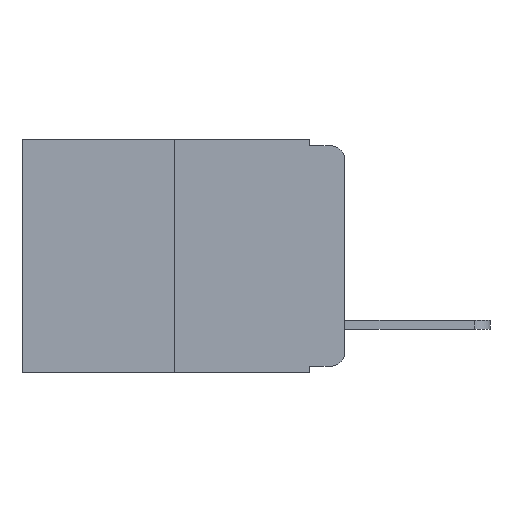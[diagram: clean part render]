
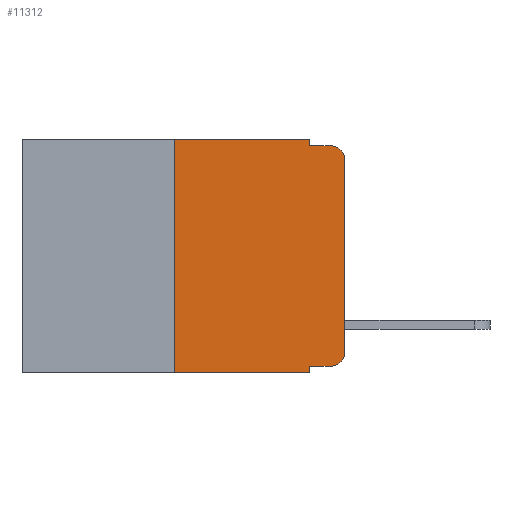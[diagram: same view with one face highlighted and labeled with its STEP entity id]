
A CAD part, left-side view. The second image highlights one B-rep face of the part: STEP entity #11312.
In plain terms, the highlighted planar face has unit normal (-1, 0, 0).
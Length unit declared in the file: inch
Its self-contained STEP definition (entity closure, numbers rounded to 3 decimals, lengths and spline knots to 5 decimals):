
#353 = CARTESIAN_POINT ( 'NONE',  ( 0., 0.25, -0.343 ) ) ;
#411 = VERTEX_POINT ( 'NONE', #8398 ) ;
#537 = DIRECTION ( 'NONE',  ( 0., 0., -1. ) ) ;
#1220 = CARTESIAN_POINT ( 'NONE',  ( 0., 0.051, 0. ) ) ;
#1526 = CARTESIAN_POINT ( 'NONE',  ( 0., 0.02, -0.01 ) ) ;
#1712 = CIRCLE ( 'NONE', #11535, 0.02 ) ;
#2218 = VERTEX_POINT ( 'NONE', #19827 ) ;
#2229 = CARTESIAN_POINT ( 'NONE',  ( 0., 0.02, -0.313 ) ) ;
#2296 = DIRECTION ( 'NONE',  ( 0., 0., -1. ) ) ;
#2300 = CARTESIAN_POINT ( 'NONE',  ( 0., 0.473, 0. ) ) ;
#2386 = LINE ( 'NONE', #2684, #10520 ) ;
#2439 = DIRECTION ( 'NONE',  ( -1., 0., 0. ) ) ;
#2684 = CARTESIAN_POINT ( 'NONE',  ( 0., 0.473, -0.343 ) ) ;
#2909 = DIRECTION ( 'NONE',  ( 0., -1., 0. ) ) ;
#3034 = VECTOR ( 'NONE', #8502, 39.37008 ) ;
#3321 = CARTESIAN_POINT ( 'NONE',  ( 0., 0., -0.313 ) ) ;
#3550 = CARTESIAN_POINT ( 'NONE',  ( 0., 0.051, -0.333 ) ) ;
#3638 = VERTEX_POINT ( 'NONE', #6824 ) ;
#3707 = PLANE ( 'NONE',  #19288 ) ;
#3893 = EDGE_CURVE ( 'NONE', #411, #12234, #6660, .T. ) ;
#4857 = CARTESIAN_POINT ( 'NONE',  ( 0., 0.02, -0.03 ) ) ;
#4941 = VERTEX_POINT ( 'NONE', #353 ) ;
#5200 = VECTOR ( 'NONE', #5649, 39.37008 ) ;
#5258 = VECTOR ( 'NONE', #20036, 39.37008 ) ;
#5277 = LINE ( 'NONE', #3550, #18646 ) ;
#5384 = LINE ( 'NONE', #5721, #6171 ) ;
#5392 = ORIENTED_EDGE ( 'NONE', *, *, #16105, .F. ) ;
#5649 = DIRECTION ( 'NONE',  ( 0., -1., 0. ) ) ;
#5721 = CARTESIAN_POINT ( 'NONE',  ( 0., 0.051, 0. ) ) ;
#5833 = CARTESIAN_POINT ( 'NONE',  ( 0., 0.25, 0. ) ) ;
#5884 = VECTOR ( 'NONE', #2909, 39.37008 ) ;
#6030 = ORIENTED_EDGE ( 'NONE', *, *, #21634, .F. ) ;
#6064 = VECTOR ( 'NONE', #8089, 39.37008 ) ;
#6171 = VECTOR ( 'NONE', #2296, 39.37008 ) ;
#6660 = LINE ( 'NONE', #19598, #5884 ) ;
#6797 = AXIS2_PLACEMENT_3D ( 'NONE', #4857, #18064, #9854 ) ;
#6824 = CARTESIAN_POINT ( 'NONE',  ( 0., 0., -0.03 ) ) ;
#7076 = CARTESIAN_POINT ( 'NONE',  ( 0., 0.473, 0. ) ) ;
#7172 = EDGE_LOOP ( 'NONE', ( #9221, #10727, #9927, #5392, #19574, #6030, #14025, #12716, #17607, #9212 ) ) ;
#7322 = EDGE_CURVE ( 'NONE', #8490, #18671, #21210, .T. ) ;
#7490 = LINE ( 'NONE', #18348, #3034 ) ;
#8089 = DIRECTION ( 'NONE',  ( 0., 0., -1. ) ) ;
#8398 = CARTESIAN_POINT ( 'NONE',  ( 0., 0.051, -0.01 ) ) ;
#8490 = VERTEX_POINT ( 'NONE', #5833 ) ;
#8502 = DIRECTION ( 'NONE',  ( 0., 0., 1. ) ) ;
#8927 = EDGE_CURVE ( 'NONE', #20630, #20075, #1712, .T. ) ;
#9088 = EDGE_CURVE ( 'NONE', #10684, #2218, #5384, .T. ) ;
#9212 = ORIENTED_EDGE ( 'NONE', *, *, #8927, .T. ) ;
#9221 = ORIENTED_EDGE ( 'NONE', *, *, #16042, .T. ) ;
#9854 = DIRECTION ( 'NONE',  ( 0., 0., -1. ) ) ;
#9927 = ORIENTED_EDGE ( 'NONE', *, *, #3893, .F. ) ;
#10251 = LINE ( 'NONE', #15062, #6064 ) ;
#10520 = VECTOR ( 'NONE', #14438, 39.37008 ) ;
#10684 = VERTEX_POINT ( 'NONE', #20153 ) ;
#10727 = ORIENTED_EDGE ( 'NONE', *, *, #12662, .T. ) ;
#11312 = ADVANCED_FACE ( 'NONE', ( #15503 ), #3707, .F. ) ;
#11458 = EDGE_CURVE ( 'NONE', #4941, #2218, #2386, .T. ) ;
#11535 = AXIS2_PLACEMENT_3D ( 'NONE', #2229, #2439, #537 ) ;
#12234 = VERTEX_POINT ( 'NONE', #1526 ) ;
#12662 = EDGE_CURVE ( 'NONE', #3638, #12234, #14805, .T. ) ;
#12716 = ORIENTED_EDGE ( 'NONE', *, *, #9088, .F. ) ;
#12935 = CARTESIAN_POINT ( 'NONE',  ( 0., 0.02, -0.333 ) ) ;
#13701 = DIRECTION ( 'NONE',  ( 1., 0., 0. ) ) ;
#13763 = DIRECTION ( 'NONE',  ( 0., -1., 0. ) ) ;
#14025 = ORIENTED_EDGE ( 'NONE', *, *, #11458, .T. ) ;
#14438 = DIRECTION ( 'NONE',  ( 0., -1., 0. ) ) ;
#14805 = CIRCLE ( 'NONE', #6797, 0.02 ) ;
#14806 = EDGE_CURVE ( 'NONE', #10684, #20630, #5277, .T. ) ;
#15000 = CARTESIAN_POINT ( 'NONE',  ( 0., 0., 0. ) ) ;
#15062 = CARTESIAN_POINT ( 'NONE',  ( 0., 0.051, 0. ) ) ;
#15421 = DIRECTION ( 'NONE',  ( 0., 0., -1. ) ) ;
#15503 = FACE_OUTER_BOUND ( 'NONE', #7172, .T. ) ;
#15763 = LINE ( 'NONE', #15000, #5258 ) ;
#16042 = EDGE_CURVE ( 'NONE', #20075, #3638, #15763, .T. ) ;
#16105 = EDGE_CURVE ( 'NONE', #18671, #411, #10251, .T. ) ;
#17607 = ORIENTED_EDGE ( 'NONE', *, *, #14806, .T. ) ;
#18064 = DIRECTION ( 'NONE',  ( -1., 0., 0. ) ) ;
#18348 = CARTESIAN_POINT ( 'NONE',  ( 0., 0.25, 0. ) ) ;
#18646 = VECTOR ( 'NONE', #13763, 39.37008 ) ;
#18671 = VERTEX_POINT ( 'NONE', #1220 ) ;
#19288 = AXIS2_PLACEMENT_3D ( 'NONE', #7076, #13701, #15421 ) ;
#19574 = ORIENTED_EDGE ( 'NONE', *, *, #7322, .F. ) ;
#19598 = CARTESIAN_POINT ( 'NONE',  ( 0., 0.051, -0.01 ) ) ;
#19827 = CARTESIAN_POINT ( 'NONE',  ( 0., 0.051, -0.343 ) ) ;
#20036 = DIRECTION ( 'NONE',  ( 0., 0., 1. ) ) ;
#20075 = VERTEX_POINT ( 'NONE', #3321 ) ;
#20153 = CARTESIAN_POINT ( 'NONE',  ( 0., 0.051, -0.333 ) ) ;
#20630 = VERTEX_POINT ( 'NONE', #12935 ) ;
#21210 = LINE ( 'NONE', #2300, #5200 ) ;
#21634 = EDGE_CURVE ( 'NONE', #4941, #8490, #7490, .T. ) ;
